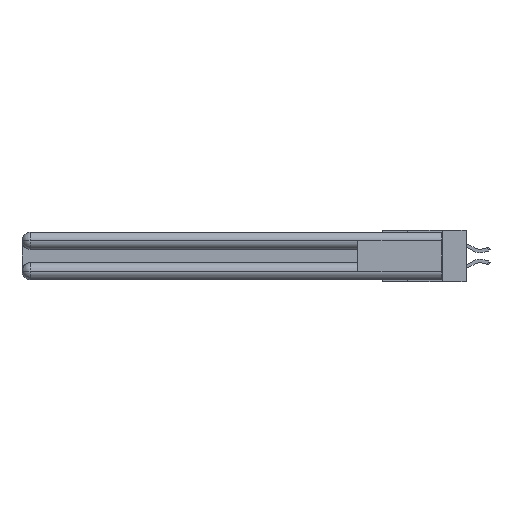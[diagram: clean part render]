
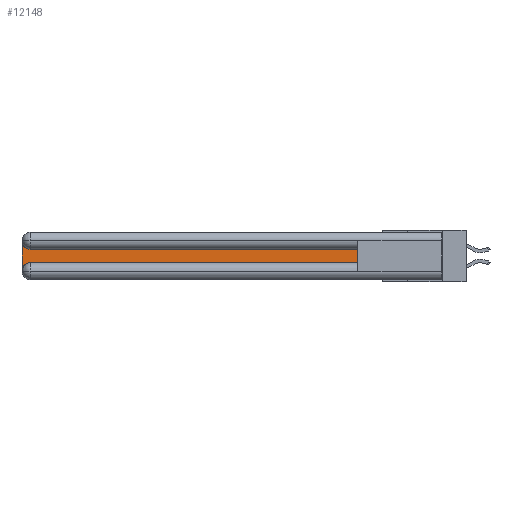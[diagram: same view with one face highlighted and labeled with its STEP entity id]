
A CAD part, left-side view. The second image highlights one B-rep face of the part: STEP entity #12148.
In plain terms, the highlighted planar face has unit normal (-1, 0, 0).
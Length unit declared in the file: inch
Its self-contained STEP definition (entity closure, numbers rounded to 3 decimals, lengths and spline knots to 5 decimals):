
#724 = CARTESIAN_POINT ( 'NONE',  ( 0.075, 3., -0.2775 ) ) ;
#1036 = DIRECTION ( 'NONE',  ( 0., 0., 1. ) ) ;
#1360 = DIRECTION ( 'NONE',  ( 0., 1., 0. ) ) ;
#1928 = DIRECTION ( 'NONE',  ( 1., 0., 0. ) ) ;
#2016 = AXIS2_PLACEMENT_3D ( 'NONE', #14665, #1928, #27922 ) ;
#3733 = CARTESIAN_POINT ( 'NONE',  ( 0.075, 2.94, -0.2175 ) ) ;
#3777 = CARTESIAN_POINT ( 'NONE',  ( 0.075, 0.6, -0.1225 ) ) ;
#4187 = EDGE_CURVE ( 'NONE', #26078, #31544, #31445, .T. ) ;
#5337 = VERTEX_POINT ( 'NONE', #33088 ) ;
#6040 = ORIENTED_EDGE ( 'NONE', *, *, #8384, .T. ) ;
#6291 = CARTESIAN_POINT ( 'NONE',  ( 0.075, 0.6, -0.2175 ) ) ;
#8280 = CARTESIAN_POINT ( 'NONE',  ( 0.075, 2.94, -0.1225 ) ) ;
#8384 = EDGE_CURVE ( 'NONE', #5337, #30774, #27528, .T. ) ;
#8812 = CARTESIAN_POINT ( 'NONE',  ( 0.075, 2.94, -0.2775 ) ) ;
#9344 = ORIENTED_EDGE ( 'NONE', *, *, #23583, .T. ) ;
#9500 = AXIS2_PLACEMENT_3D ( 'NONE', #8812, #14004, #27186 ) ;
#9667 = VECTOR ( 'NONE', #1360, 39.37008 ) ;
#10971 = VECTOR ( 'NONE', #24124, 39.37008 ) ;
#11453 = CARTESIAN_POINT ( 'NONE',  ( 0.075, 3., -0.2175 ) ) ;
#11872 = VECTOR ( 'NONE', #1036, 39.37008 ) ;
#12133 = CIRCLE ( 'NONE', #23723, 0.06 ) ;
#12148 = ADVANCED_FACE ( 'NONE', ( #31340 ), #22571, .F. ) ;
#13787 = LINE ( 'NONE', #11453, #10971 ) ;
#14004 = DIRECTION ( 'NONE',  ( 1., 0., 0. ) ) ;
#14665 = CARTESIAN_POINT ( 'NONE',  ( 0.075, 3., -0.1225 ) ) ;
#16600 = ORIENTED_EDGE ( 'NONE', *, *, #24100, .T. ) ;
#18080 = ORIENTED_EDGE ( 'NONE', *, *, #4187, .T. ) ;
#20808 = DIRECTION ( 'NONE',  ( 1., 0., 0. ) ) ;
#22175 = EDGE_CURVE ( 'NONE', #27437, #5337, #28936, .T. ) ;
#22571 = PLANE ( 'NONE',  #2016 ) ;
#23263 = CARTESIAN_POINT ( 'NONE',  ( 0.075, 2.94, -0.0625 ) ) ;
#23583 = EDGE_CURVE ( 'NONE', #23644, #26078, #13787, .T. ) ;
#23644 = VERTEX_POINT ( 'NONE', #29368 ) ;
#23723 = AXIS2_PLACEMENT_3D ( 'NONE', #23263, #20808, #25901 ) ;
#23899 = EDGE_CURVE ( 'NONE', #31544, #27437, #32876, .T. ) ;
#24100 = EDGE_CURVE ( 'NONE', #30774, #23644, #12133, .T. ) ;
#24124 = DIRECTION ( 'NONE',  ( 0., 0., -1. ) ) ;
#24413 = ORIENTED_EDGE ( 'NONE', *, *, #22175, .T. ) ;
#25901 = DIRECTION ( 'NONE',  ( 0., 0., -1. ) ) ;
#25937 = VECTOR ( 'NONE', #30676, 39.37008 ) ;
#26078 = VERTEX_POINT ( 'NONE', #724 ) ;
#26595 = ORIENTED_EDGE ( 'NONE', *, *, #23899, .T. ) ;
#27186 = DIRECTION ( 'NONE',  ( 0., 0., -1. ) ) ;
#27437 = VERTEX_POINT ( 'NONE', #31190 ) ;
#27528 = LINE ( 'NONE', #3777, #9667 ) ;
#27922 = DIRECTION ( 'NONE',  ( 0., 0., -1. ) ) ;
#27953 = CARTESIAN_POINT ( 'NONE',  ( 0.075, 0.6, -0.2175 ) ) ;
#28936 = LINE ( 'NONE', #6291, #11872 ) ;
#29368 = CARTESIAN_POINT ( 'NONE',  ( 0.075, 3., -0.0625 ) ) ;
#30676 = DIRECTION ( 'NONE',  ( 0., -1., 0. ) ) ;
#30774 = VERTEX_POINT ( 'NONE', #8280 ) ;
#31190 = CARTESIAN_POINT ( 'NONE',  ( 0.075, 0.6, -0.2175 ) ) ;
#31284 = EDGE_LOOP ( 'NONE', ( #6040, #16600, #9344, #18080, #26595, #24413 ) ) ;
#31340 = FACE_OUTER_BOUND ( 'NONE', #31284, .T. ) ;
#31445 = CIRCLE ( 'NONE', #9500, 0.06 ) ;
#31544 = VERTEX_POINT ( 'NONE', #3733 ) ;
#32876 = LINE ( 'NONE', #27953, #25937 ) ;
#33088 = CARTESIAN_POINT ( 'NONE',  ( 0.075, 0.6, -0.1225 ) ) ;
